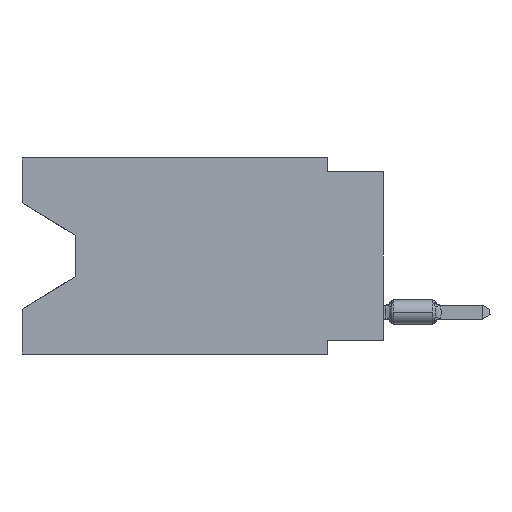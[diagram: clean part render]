
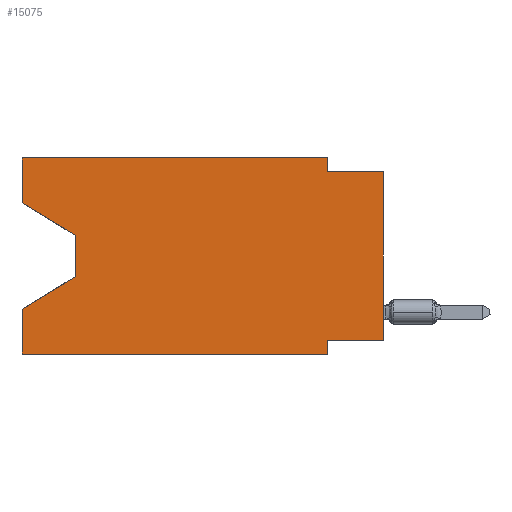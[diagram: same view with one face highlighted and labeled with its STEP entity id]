
A CAD part, left-side view. The second image highlights one B-rep face of the part: STEP entity #15075.
In plain terms, the highlighted planar face has unit normal (-1, 0, 0).
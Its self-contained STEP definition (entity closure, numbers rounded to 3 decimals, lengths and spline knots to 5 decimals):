
#927 = ORIENTED_EDGE ( 'NONE', *, *, #17718, .T. ) ;
#2863 = LINE ( 'NONE', #39800, #22087 ) ;
#2993 = VECTOR ( 'NONE', #32245, 39.37008 ) ;
#4731 = LINE ( 'NONE', #13163, #43676 ) ;
#4965 = VERTEX_POINT ( 'NONE', #42804 ) ;
#5007 = DIRECTION ( 'NONE',  ( 0., 0., -1. ) ) ;
#5346 = EDGE_CURVE ( 'NONE', #53146, #47326, #4731, .T. ) ;
#5832 = CARTESIAN_POINT ( 'NONE',  ( 0., 0., -0.325 ) ) ;
#7671 = EDGE_CURVE ( 'NONE', #37433, #8771, #15825, .T. ) ;
#7945 = CARTESIAN_POINT ( 'NONE',  ( 0., 0.645, 0. ) ) ;
#8771 = VERTEX_POINT ( 'NONE', #7945 ) ;
#10482 = VECTOR ( 'NONE', #48824, 39.37008 ) ;
#11382 = DIRECTION ( 'NONE',  ( 1., 0., 0. ) ) ;
#13122 = ORIENTED_EDGE ( 'NONE', *, *, #5346, .F. ) ;
#13163 = CARTESIAN_POINT ( 'NONE',  ( 0., 0.1, 0. ) ) ;
#14756 = VERTEX_POINT ( 'NONE', #50239 ) ;
#14925 = PLANE ( 'NONE',  #50146 ) ;
#15075 = ADVANCED_FACE ( 'NONE', ( #23056 ), #14925, .F. ) ;
#15612 = CARTESIAN_POINT ( 'NONE',  ( 0., 0.645, -0.26975 ) ) ;
#15825 = LINE ( 'NONE', #23707, #27357 ) ;
#16033 = DIRECTION ( 'NONE',  ( 0., 0.855, -0.519 ) ) ;
#16537 = CARTESIAN_POINT ( 'NONE',  ( 0., 0.645, -0.35 ) ) ;
#17173 = LINE ( 'NONE', #46487, #47310 ) ;
#17464 = CARTESIAN_POINT ( 'NONE',  ( 0., 0., 0. ) ) ;
#17718 = EDGE_CURVE ( 'NONE', #30738, #40561, #28553, .T. ) ;
#17784 = DIRECTION ( 'NONE',  ( 0., 1., 0. ) ) ;
#18288 = EDGE_CURVE ( 'NONE', #30148, #38855, #30282, .T. ) ;
#18392 = ORIENTED_EDGE ( 'NONE', *, *, #50570, .F. ) ;
#18417 = LINE ( 'NONE', #52108, #50087 ) ;
#19415 = DIRECTION ( 'NONE',  ( 0., 0., -1. ) ) ;
#19862 = CARTESIAN_POINT ( 'NONE',  ( 0., 0.55, -0.212 ) ) ;
#20022 = EDGE_LOOP ( 'NONE', ( #21368, #23068, #927, #33162, #28112, #20908, #26901, #45977, #18392, #13122, #46341, #23402 ) ) ;
#20293 = LINE ( 'NONE', #20846, #10482 ) ;
#20846 = CARTESIAN_POINT ( 'NONE',  ( 0., 0.645, -0.08025 ) ) ;
#20908 = ORIENTED_EDGE ( 'NONE', *, *, #21123, .F. ) ;
#21123 = EDGE_CURVE ( 'NONE', #38855, #4965, #41528, .T. ) ;
#21368 = ORIENTED_EDGE ( 'NONE', *, *, #48365, .T. ) ;
#22087 = VECTOR ( 'NONE', #19415, 39.37008 ) ;
#23056 = FACE_OUTER_BOUND ( 'NONE', #20022, .T. ) ;
#23068 = ORIENTED_EDGE ( 'NONE', *, *, #40656, .T. ) ;
#23402 = ORIENTED_EDGE ( 'NONE', *, *, #7671, .F. ) ;
#23707 = CARTESIAN_POINT ( 'NONE',  ( 0., 0.645, 0. ) ) ;
#24771 = EDGE_CURVE ( 'NONE', #8771, #53146, #28877, .T. ) ;
#26443 = VECTOR ( 'NONE', #45968, 39.37008 ) ;
#26901 = ORIENTED_EDGE ( 'NONE', *, *, #18288, .F. ) ;
#27357 = VECTOR ( 'NONE', #28327, 39.37008 ) ;
#28112 = ORIENTED_EDGE ( 'NONE', *, *, #44901, .T. ) ;
#28327 = DIRECTION ( 'NONE',  ( 0., 0., 1. ) ) ;
#28553 = LINE ( 'NONE', #19862, #36132 ) ;
#28877 = LINE ( 'NONE', #37300, #26443 ) ;
#30148 = VERTEX_POINT ( 'NONE', #38415 ) ;
#30282 = LINE ( 'NONE', #5832, #37895 ) ;
#30498 = DIRECTION ( 'NONE',  ( 0., 0., 1. ) ) ;
#30738 = VERTEX_POINT ( 'NONE', #52470 ) ;
#32245 = DIRECTION ( 'NONE',  ( 0., 0., 1. ) ) ;
#33162 = ORIENTED_EDGE ( 'NONE', *, *, #40120, .F. ) ;
#33654 = CARTESIAN_POINT ( 'NONE',  ( 0., 0.645, -0.08025 ) ) ;
#33780 = LINE ( 'NONE', #17464, #35914 ) ;
#33903 = VERTEX_POINT ( 'NONE', #16537 ) ;
#34853 = CARTESIAN_POINT ( 'NONE',  ( 0., 0.1, -0.025 ) ) ;
#35914 = VECTOR ( 'NONE', #30498, 39.37008 ) ;
#36132 = VECTOR ( 'NONE', #16033, 39.37008 ) ;
#37300 = CARTESIAN_POINT ( 'NONE',  ( 0., 0.645, 0. ) ) ;
#37433 = VERTEX_POINT ( 'NONE', #33654 ) ;
#37801 = DIRECTION ( 'NONE',  ( 0., -1., 0. ) ) ;
#37895 = VECTOR ( 'NONE', #17784, 39.37008 ) ;
#38415 = CARTESIAN_POINT ( 'NONE',  ( 0., 0., -0.325 ) ) ;
#38855 = VERTEX_POINT ( 'NONE', #39679 ) ;
#39120 = EDGE_CURVE ( 'NONE', #30148, #14756, #33780, .T. ) ;
#39439 = CARTESIAN_POINT ( 'NONE',  ( 0., 0.1, 0. ) ) ;
#39625 = DIRECTION ( 'NONE',  ( 0., 0., -1. ) ) ;
#39679 = CARTESIAN_POINT ( 'NONE',  ( 0., 0.1, -0.325 ) ) ;
#39800 = CARTESIAN_POINT ( 'NONE',  ( 0., 0.55, -0.138 ) ) ;
#40120 = EDGE_CURVE ( 'NONE', #33903, #40561, #46930, .T. ) ;
#40130 = DIRECTION ( 'NONE',  ( 0., -1., 0. ) ) ;
#40559 = CARTESIAN_POINT ( 'NONE',  ( 0., 0.55, -0.138 ) ) ;
#40561 = VERTEX_POINT ( 'NONE', #15612 ) ;
#40656 = EDGE_CURVE ( 'NONE', #51797, #30738, #2863, .T. ) ;
#41528 = LINE ( 'NONE', #49422, #49433 ) ;
#42804 = CARTESIAN_POINT ( 'NONE',  ( 0., 0.1, -0.35 ) ) ;
#43676 = VECTOR ( 'NONE', #5007, 39.37008 ) ;
#44901 = EDGE_CURVE ( 'NONE', #33903, #4965, #18417, .T. ) ;
#45968 = DIRECTION ( 'NONE',  ( 0., -1., 0. ) ) ;
#45977 = ORIENTED_EDGE ( 'NONE', *, *, #39120, .T. ) ;
#46341 = ORIENTED_EDGE ( 'NONE', *, *, #24771, .F. ) ;
#46487 = CARTESIAN_POINT ( 'NONE',  ( 0., 0., -0.025 ) ) ;
#46930 = LINE ( 'NONE', #49072, #2993 ) ;
#47310 = VECTOR ( 'NONE', #37801, 39.37008 ) ;
#47326 = VERTEX_POINT ( 'NONE', #34853 ) ;
#48365 = EDGE_CURVE ( 'NONE', #37433, #51797, #20293, .T. ) ;
#48824 = DIRECTION ( 'NONE',  ( 0., -0.855, -0.519 ) ) ;
#49072 = CARTESIAN_POINT ( 'NONE',  ( 0., 0.645, 0. ) ) ;
#49422 = CARTESIAN_POINT ( 'NONE',  ( 0., 0.1, -0.35 ) ) ;
#49433 = VECTOR ( 'NONE', #50942, 39.37008 ) ;
#50087 = VECTOR ( 'NONE', #40130, 39.37008 ) ;
#50146 = AXIS2_PLACEMENT_3D ( 'NONE', #52391, #11382, #39625 ) ;
#50239 = CARTESIAN_POINT ( 'NONE',  ( 0., 0., -0.025 ) ) ;
#50570 = EDGE_CURVE ( 'NONE', #47326, #14756, #17173, .T. ) ;
#50942 = DIRECTION ( 'NONE',  ( 0., 0., -1. ) ) ;
#51797 = VERTEX_POINT ( 'NONE', #40559 ) ;
#52108 = CARTESIAN_POINT ( 'NONE',  ( 0., 0.645, -0.35 ) ) ;
#52391 = CARTESIAN_POINT ( 'NONE',  ( 0., 0.645, 0. ) ) ;
#52470 = CARTESIAN_POINT ( 'NONE',  ( 0., 0.55, -0.212 ) ) ;
#53146 = VERTEX_POINT ( 'NONE', #39439 ) ;
